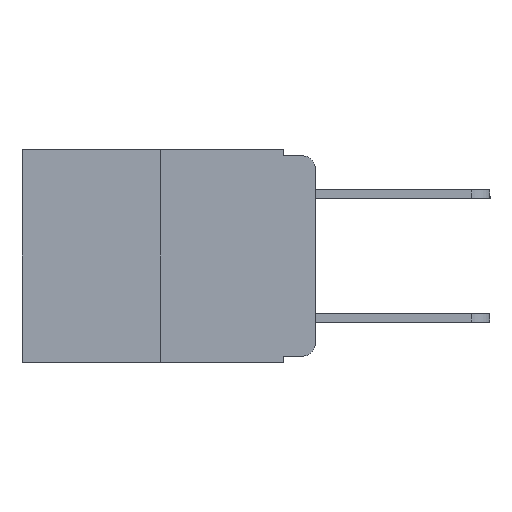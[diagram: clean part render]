
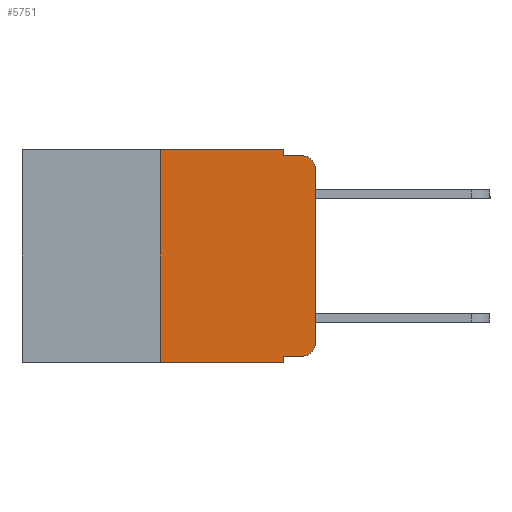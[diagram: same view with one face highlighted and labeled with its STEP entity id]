
A CAD part, left-side view. The second image highlights one B-rep face of the part: STEP entity #5751.
In plain terms, the highlighted planar face has unit normal (-1, 0, 0).
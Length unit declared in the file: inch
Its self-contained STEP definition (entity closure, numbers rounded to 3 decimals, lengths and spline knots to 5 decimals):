
#169 = LINE ( 'NONE', #1084, #16044 ) ;
#399 = CARTESIAN_POINT ( 'NONE',  ( 0., 0., -0.313 ) ) ;
#522 = VERTEX_POINT ( 'NONE', #9470 ) ;
#1084 = CARTESIAN_POINT ( 'NONE',  ( 0., 0.473, -0.343 ) ) ;
#1495 = VECTOR ( 'NONE', #4252, 39.37008 ) ;
#1665 = DIRECTION ( 'NONE',  ( 0., -1., 0. ) ) ;
#1976 = CARTESIAN_POINT ( 'NONE',  ( 0., 0.051, -0.333 ) ) ;
#2022 = VERTEX_POINT ( 'NONE', #11183 ) ;
#2584 = VERTEX_POINT ( 'NONE', #9747 ) ;
#2668 = VERTEX_POINT ( 'NONE', #399 ) ;
#2706 = EDGE_CURVE ( 'NONE', #6036, #522, #169, .T. ) ;
#2779 = CARTESIAN_POINT ( 'NONE',  ( 0., 0.473, 0. ) ) ;
#2840 = EDGE_CURVE ( 'NONE', #15682, #2022, #17456, .T. ) ;
#3029 = ORIENTED_EDGE ( 'NONE', *, *, #10146, .T. ) ;
#3172 = VERTEX_POINT ( 'NONE', #18537 ) ;
#3310 = ORIENTED_EDGE ( 'NONE', *, *, #5071, .T. ) ;
#3350 = ORIENTED_EDGE ( 'NONE', *, *, #4022, .F. ) ;
#3356 = LINE ( 'NONE', #5898, #11024 ) ;
#3396 = ORIENTED_EDGE ( 'NONE', *, *, #2840, .F. ) ;
#3542 = ORIENTED_EDGE ( 'NONE', *, *, #13231, .F. ) ;
#3625 = VERTEX_POINT ( 'NONE', #18719 ) ;
#3712 = DIRECTION ( 'NONE',  ( 0., -1., 0. ) ) ;
#3769 = PLANE ( 'NONE',  #12550 ) ;
#4022 = EDGE_CURVE ( 'NONE', #2022, #3172, #4438, .T. ) ;
#4252 = DIRECTION ( 'NONE',  ( 0., 0., 1. ) ) ;
#4261 = CARTESIAN_POINT ( 'NONE',  ( 0., 0.25, 0. ) ) ;
#4357 = ORIENTED_EDGE ( 'NONE', *, *, #18031, .F. ) ;
#4438 = LINE ( 'NONE', #13357, #19196 ) ;
#4587 = ORIENTED_EDGE ( 'NONE', *, *, #2706, .T. ) ;
#5071 = EDGE_CURVE ( 'NONE', #3625, #3172, #5961, .T. ) ;
#5109 = DIRECTION ( 'NONE',  ( 0., 0., -1. ) ) ;
#5339 = DIRECTION ( 'NONE',  ( 0., 0., -1. ) ) ;
#5517 = ORIENTED_EDGE ( 'NONE', *, *, #11478, .F. ) ;
#5678 = ORIENTED_EDGE ( 'NONE', *, *, #10505, .T. ) ;
#5751 = ADVANCED_FACE ( 'NONE', ( #6166 ), #3769, .F. ) ;
#5890 = ORIENTED_EDGE ( 'NONE', *, *, #8579, .T. ) ;
#5898 = CARTESIAN_POINT ( 'NONE',  ( 0., 0.051, 0. ) ) ;
#5961 = CIRCLE ( 'NONE', #11649, 0.02 ) ;
#6036 = VERTEX_POINT ( 'NONE', #16442 ) ;
#6166 = FACE_OUTER_BOUND ( 'NONE', #18324, .T. ) ;
#6599 = LINE ( 'NONE', #10045, #14408 ) ;
#7093 = DIRECTION ( 'NONE',  ( 0., -1., 0. ) ) ;
#7410 = CARTESIAN_POINT ( 'NONE',  ( 0., 0.051, 0. ) ) ;
#7428 = DIRECTION ( 'NONE',  ( 0., 0., -1. ) ) ;
#7710 = CARTESIAN_POINT ( 'NONE',  ( 0., 0.25, 0. ) ) ;
#7926 = VECTOR ( 'NONE', #9170, 39.37008 ) ;
#8395 = LINE ( 'NONE', #7710, #7926 ) ;
#8579 = EDGE_CURVE ( 'NONE', #15023, #2668, #14341, .T. ) ;
#9170 = DIRECTION ( 'NONE',  ( 0., 0., 1. ) ) ;
#9306 = DIRECTION ( 'NONE',  ( 0., 0., -1. ) ) ;
#9470 = CARTESIAN_POINT ( 'NONE',  ( 0., 0.051, -0.343 ) ) ;
#9747 = CARTESIAN_POINT ( 'NONE',  ( 0., 0.051, -0.333 ) ) ;
#9952 = VECTOR ( 'NONE', #3712, 39.37008 ) ;
#10045 = CARTESIAN_POINT ( 'NONE',  ( 0., 0.473, 0. ) ) ;
#10146 = EDGE_CURVE ( 'NONE', #2668, #3625, #13808, .T. ) ;
#10408 = LINE ( 'NONE', #1976, #9952 ) ;
#10505 = EDGE_CURVE ( 'NONE', #2584, #15023, #10408, .T. ) ;
#10694 = DIRECTION ( 'NONE',  ( -1., 0., 0. ) ) ;
#10872 = CARTESIAN_POINT ( 'NONE',  ( 0., 0.051, 0. ) ) ;
#11024 = VECTOR ( 'NONE', #7428, 39.37008 ) ;
#11124 = CARTESIAN_POINT ( 'NONE',  ( 0., 0.02, -0.313 ) ) ;
#11183 = CARTESIAN_POINT ( 'NONE',  ( 0., 0.051, -0.01 ) ) ;
#11478 = EDGE_CURVE ( 'NONE', #2584, #522, #3356, .T. ) ;
#11649 = AXIS2_PLACEMENT_3D ( 'NONE', #17754, #17732, #5339 ) ;
#12550 = AXIS2_PLACEMENT_3D ( 'NONE', #2779, #12908, #13926 ) ;
#12908 = DIRECTION ( 'NONE',  ( 1., 0., 0. ) ) ;
#13231 = EDGE_CURVE ( 'NONE', #16157, #15682, #6599, .T. ) ;
#13357 = CARTESIAN_POINT ( 'NONE',  ( 0., 0.051, -0.01 ) ) ;
#13808 = LINE ( 'NONE', #17331, #1495 ) ;
#13832 = VECTOR ( 'NONE', #5109, 39.37008 ) ;
#13926 = DIRECTION ( 'NONE',  ( 0., 0., -1. ) ) ;
#14341 = CIRCLE ( 'NONE', #19132, 0.02 ) ;
#14408 = VECTOR ( 'NONE', #7093, 39.37008 ) ;
#15023 = VERTEX_POINT ( 'NONE', #17001 ) ;
#15682 = VERTEX_POINT ( 'NONE', #10872 ) ;
#16044 = VECTOR ( 'NONE', #1665, 39.37008 ) ;
#16157 = VERTEX_POINT ( 'NONE', #4261 ) ;
#16442 = CARTESIAN_POINT ( 'NONE',  ( 0., 0.25, -0.343 ) ) ;
#17001 = CARTESIAN_POINT ( 'NONE',  ( 0., 0.02, -0.333 ) ) ;
#17331 = CARTESIAN_POINT ( 'NONE',  ( 0., 0., 0. ) ) ;
#17456 = LINE ( 'NONE', #7410, #13832 ) ;
#17645 = DIRECTION ( 'NONE',  ( 0., -1., 0. ) ) ;
#17732 = DIRECTION ( 'NONE',  ( -1., 0., 0. ) ) ;
#17754 = CARTESIAN_POINT ( 'NONE',  ( 0., 0.02, -0.03 ) ) ;
#18031 = EDGE_CURVE ( 'NONE', #6036, #16157, #8395, .T. ) ;
#18324 = EDGE_LOOP ( 'NONE', ( #3029, #3310, #3350, #3396, #3542, #4357, #4587, #5517, #5678, #5890 ) ) ;
#18537 = CARTESIAN_POINT ( 'NONE',  ( 0., 0.02, -0.01 ) ) ;
#18719 = CARTESIAN_POINT ( 'NONE',  ( 0., 0., -0.03 ) ) ;
#19132 = AXIS2_PLACEMENT_3D ( 'NONE', #11124, #10694, #9306 ) ;
#19196 = VECTOR ( 'NONE', #17645, 39.37008 ) ;
